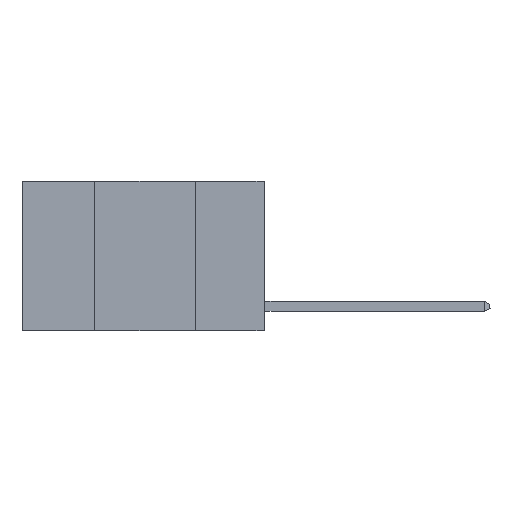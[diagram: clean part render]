
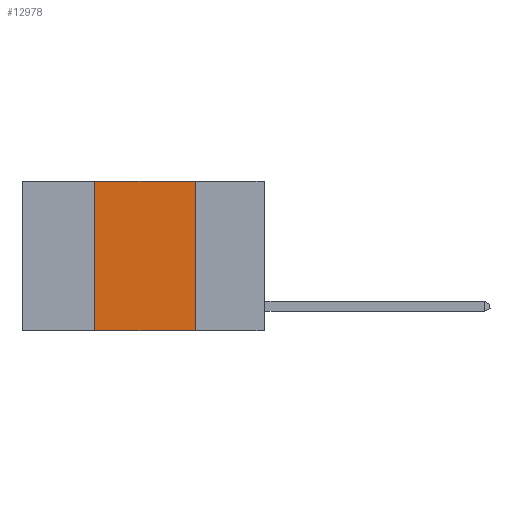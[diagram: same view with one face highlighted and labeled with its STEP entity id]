
A CAD part, left-side view. The second image highlights one B-rep face of the part: STEP entity #12978.
In plain terms, the highlighted planar face has unit normal (-1, 0, 0).
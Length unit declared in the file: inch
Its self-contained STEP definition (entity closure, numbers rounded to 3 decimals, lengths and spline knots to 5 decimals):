
#2875 = VECTOR ( 'NONE', #4553, 39.37008 ) ;
#2877 = ORIENTED_EDGE ( 'NONE', *, *, #16856, .F. ) ;
#3576 = LINE ( 'NONE', #11189, #2875 ) ;
#4553 = DIRECTION ( 'NONE',  ( 0., 0., 1. ) ) ;
#5607 = LINE ( 'NONE', #27907, #23379 ) ;
#6620 = CARTESIAN_POINT ( 'NONE',  ( 0., 0.42, 0. ) ) ;
#7534 = VERTEX_POINT ( 'NONE', #23911 ) ;
#7986 = PLANE ( 'NONE',  #20666 ) ;
#9175 = ORIENTED_EDGE ( 'NONE', *, *, #15305, .F. ) ;
#10243 = DIRECTION ( 'NONE',  ( 0., 0., -1. ) ) ;
#11189 = CARTESIAN_POINT ( 'NONE',  ( 0., 0.42, 0. ) ) ;
#12296 = EDGE_CURVE ( 'NONE', #13486, #7534, #5607, .T. ) ;
#12382 = DIRECTION ( 'NONE',  ( 0., -1., 0. ) ) ;
#12978 = ADVANCED_FACE ( 'NONE', ( #17809 ), #7986, .F. ) ;
#13296 = DIRECTION ( 'NONE',  ( 0., 0., -1. ) ) ;
#13426 = EDGE_LOOP ( 'NONE', ( #23826, #2877, #9175, #15139 ) ) ;
#13486 = VERTEX_POINT ( 'NONE', #16362 ) ;
#14194 = VECTOR ( 'NONE', #13296, 39.37008 ) ;
#15139 = ORIENTED_EDGE ( 'NONE', *, *, #12296, .T. ) ;
#15305 = EDGE_CURVE ( 'NONE', #13486, #22782, #3576, .T. ) ;
#16362 = CARTESIAN_POINT ( 'NONE',  ( 0., 0.42, -0.37 ) ) ;
#16856 = EDGE_CURVE ( 'NONE', #22782, #22958, #19551, .T. ) ;
#17809 = FACE_OUTER_BOUND ( 'NONE', #13426, .T. ) ;
#18967 = DIRECTION ( 'NONE',  ( 0., -1., 0. ) ) ;
#19051 = EDGE_CURVE ( 'NONE', #22958, #7534, #20806, .T. ) ;
#19132 = CARTESIAN_POINT ( 'NONE',  ( 0., 0.6, 0. ) ) ;
#19551 = LINE ( 'NONE', #27953, #24768 ) ;
#20566 = CARTESIAN_POINT ( 'NONE',  ( 0., 0.17, 0. ) ) ;
#20666 = AXIS2_PLACEMENT_3D ( 'NONE', #19132, #23604, #10243 ) ;
#20806 = LINE ( 'NONE', #22201, #14194 ) ;
#22201 = CARTESIAN_POINT ( 'NONE',  ( 0., 0.17, 0. ) ) ;
#22782 = VERTEX_POINT ( 'NONE', #6620 ) ;
#22958 = VERTEX_POINT ( 'NONE', #20566 ) ;
#23379 = VECTOR ( 'NONE', #18967, 39.37008 ) ;
#23604 = DIRECTION ( 'NONE',  ( 1., 0., 0. ) ) ;
#23826 = ORIENTED_EDGE ( 'NONE', *, *, #19051, .F. ) ;
#23911 = CARTESIAN_POINT ( 'NONE',  ( 0., 0.17, -0.37 ) ) ;
#24768 = VECTOR ( 'NONE', #12382, 39.37008 ) ;
#27907 = CARTESIAN_POINT ( 'NONE',  ( 0., 0.6, -0.37 ) ) ;
#27953 = CARTESIAN_POINT ( 'NONE',  ( 0., 0.6, 0. ) ) ;
